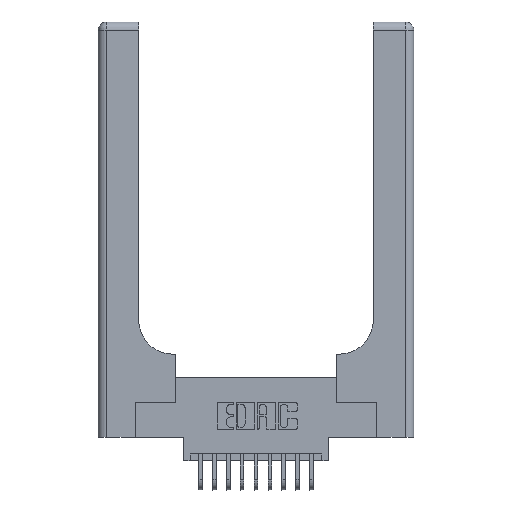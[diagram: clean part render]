
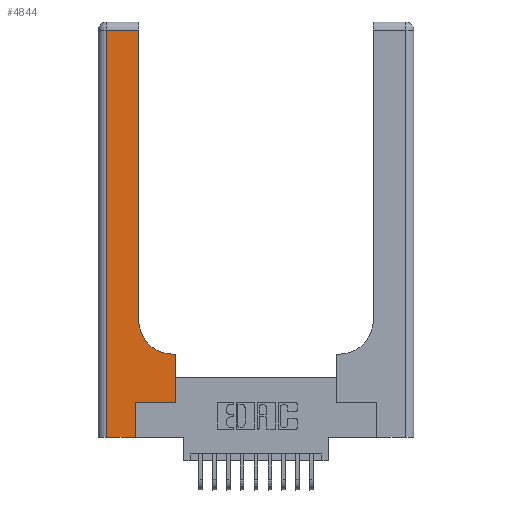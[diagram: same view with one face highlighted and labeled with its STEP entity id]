
A CAD part, top view. The second image highlights one B-rep face of the part: STEP entity #4844.
In plain terms, the highlighted planar face has unit normal (0, 0, 1).
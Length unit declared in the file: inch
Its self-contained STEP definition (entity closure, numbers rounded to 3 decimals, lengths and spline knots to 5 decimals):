
#27 = CARTESIAN_POINT ( 'NONE',  ( 0.2915, 2.94, 0.37 ) ) ;
#61 = DIRECTION ( 'NONE',  ( 0., 1., 0. ) ) ;
#300 = LINE ( 'NONE', #10796, #16571 ) ;
#415 = ORIENTED_EDGE ( 'NONE', *, *, #14892, .T. ) ;
#461 = DIRECTION ( 'NONE',  ( -1., 0., 0. ) ) ;
#616 = VECTOR ( 'NONE', #9260, 39.37008 ) ;
#671 = LINE ( 'NONE', #7835, #15627 ) ;
#719 = CARTESIAN_POINT ( 'NONE',  ( 0.5415, 0.6, 0.37 ) ) ;
#1242 = CARTESIAN_POINT ( 'NONE',  ( 0.269, 0., 0.37 ) ) ;
#1397 = CARTESIAN_POINT ( 'NONE',  ( 0.269, 0.25, 0.37 ) ) ;
#1563 = AXIS2_PLACEMENT_3D ( 'NONE', #11210, #4043, #2668 ) ;
#1673 = LINE ( 'NONE', #11323, #16840 ) ;
#1969 = CARTESIAN_POINT ( 'NONE',  ( 0.5585, 0.6, 0.37 ) ) ;
#2200 = DIRECTION ( 'NONE',  ( 0., 0., -1. ) ) ;
#2320 = CARTESIAN_POINT ( 'NONE',  ( 0.5415, 0.85, 0.37 ) ) ;
#2668 = DIRECTION ( 'NONE',  ( -1., 0., 0. ) ) ;
#2923 = CARTESIAN_POINT ( 'NONE',  ( 0.269, 0., 0.37 ) ) ;
#2958 = EDGE_CURVE ( 'NONE', #10657, #16845, #16515, .T. ) ;
#4043 = DIRECTION ( 'NONE',  ( 0., 0., -1. ) ) ;
#4255 = DIRECTION ( 'NONE',  ( -1., 0., 0. ) ) ;
#4281 = VERTEX_POINT ( 'NONE', #13822 ) ;
#4439 = LINE ( 'NONE', #8953, #616 ) ;
#4489 = ORIENTED_EDGE ( 'NONE', *, *, #18463, .T. ) ;
#4693 = LINE ( 'NONE', #1397, #8007 ) ;
#4844 = ADVANCED_FACE ( 'NONE', ( #7493 ), #15517, .F. ) ;
#5193 = DIRECTION ( 'NONE',  ( 1., 0., 0. ) ) ;
#5352 = VECTOR ( 'NONE', #461, 39.37008 ) ;
#5549 = CARTESIAN_POINT ( 'NONE',  ( 0.269, 0.25, 0.37 ) ) ;
#6067 = EDGE_CURVE ( 'NONE', #6499, #9241, #13495, .T. ) ;
#6171 = EDGE_LOOP ( 'NONE', ( #14357, #415, #17173, #10619, #13718, #17838, #4489, #11996, #8521 ) ) ;
#6417 = EDGE_CURVE ( 'NONE', #16845, #16767, #11688, .T. ) ;
#6499 = VERTEX_POINT ( 'NONE', #2923 ) ;
#7059 = VERTEX_POINT ( 'NONE', #16947 ) ;
#7493 = FACE_OUTER_BOUND ( 'NONE', #6171, .T. ) ;
#7745 = VECTOR ( 'NONE', #4255, 39.37008 ) ;
#7835 = CARTESIAN_POINT ( 'NONE',  ( 0., 0., 0.37 ) ) ;
#8007 = VECTOR ( 'NONE', #16933, 39.37008 ) ;
#8521 = ORIENTED_EDGE ( 'NONE', *, *, #6417, .T. ) ;
#8706 = CARTESIAN_POINT ( 'NONE',  ( 0.06, 2.94, 0.37 ) ) ;
#8884 = EDGE_CURVE ( 'NONE', #14968, #7059, #1673, .T. ) ;
#8953 = CARTESIAN_POINT ( 'NONE',  ( 0.2915, 3., 0.37 ) ) ;
#9241 = VERTEX_POINT ( 'NONE', #5549 ) ;
#9260 = DIRECTION ( 'NONE',  ( 0., 1., 0. ) ) ;
#10619 = ORIENTED_EDGE ( 'NONE', *, *, #11427, .T. ) ;
#10657 = VERTEX_POINT ( 'NONE', #1969 ) ;
#10796 = CARTESIAN_POINT ( 'NONE',  ( 0.5585, 0.25, 0.37 ) ) ;
#11210 = CARTESIAN_POINT ( 'NONE',  ( 0., 3., 0.37 ) ) ;
#11323 = CARTESIAN_POINT ( 'NONE',  ( 0.06, 3., 0.37 ) ) ;
#11427 = EDGE_CURVE ( 'NONE', #7059, #6499, #671, .T. ) ;
#11688 = CIRCLE ( 'NONE', #14840, 0.25 ) ;
#11996 = ORIENTED_EDGE ( 'NONE', *, *, #2958, .T. ) ;
#12262 = EDGE_CURVE ( 'NONE', #9241, #4281, #4693, .T. ) ;
#12531 = CARTESIAN_POINT ( 'NONE',  ( 0., 2.94, 0.37 ) ) ;
#12570 = VERTEX_POINT ( 'NONE', #27 ) ;
#13331 = EDGE_CURVE ( 'NONE', #16767, #12570, #4439, .T. ) ;
#13495 = LINE ( 'NONE', #1242, #17522 ) ;
#13718 = ORIENTED_EDGE ( 'NONE', *, *, #6067, .T. ) ;
#13822 = CARTESIAN_POINT ( 'NONE',  ( 0.5585, 0.25, 0.37 ) ) ;
#13823 = CARTESIAN_POINT ( 'NONE',  ( 0.2915, 0.85, 0.37 ) ) ;
#14249 = DIRECTION ( 'NONE',  ( 0., -1., 0. ) ) ;
#14357 = ORIENTED_EDGE ( 'NONE', *, *, #13331, .T. ) ;
#14457 = LINE ( 'NONE', #12531, #7745 ) ;
#14840 = AXIS2_PLACEMENT_3D ( 'NONE', #2320, #2200, #5193 ) ;
#14892 = EDGE_CURVE ( 'NONE', #12570, #14968, #14457, .T. ) ;
#14968 = VERTEX_POINT ( 'NONE', #8706 ) ;
#15517 = PLANE ( 'NONE',  #1563 ) ;
#15627 = VECTOR ( 'NONE', #16583, 39.37008 ) ;
#16515 = LINE ( 'NONE', #17560, #5352 ) ;
#16571 = VECTOR ( 'NONE', #18116, 39.37008 ) ;
#16583 = DIRECTION ( 'NONE',  ( 1., 0., 0. ) ) ;
#16767 = VERTEX_POINT ( 'NONE', #13823 ) ;
#16840 = VECTOR ( 'NONE', #14249, 39.37008 ) ;
#16845 = VERTEX_POINT ( 'NONE', #719 ) ;
#16933 = DIRECTION ( 'NONE',  ( 1., 0., 0. ) ) ;
#16947 = CARTESIAN_POINT ( 'NONE',  ( 0.06, 0., 0.37 ) ) ;
#17173 = ORIENTED_EDGE ( 'NONE', *, *, #8884, .T. ) ;
#17522 = VECTOR ( 'NONE', #61, 39.37008 ) ;
#17560 = CARTESIAN_POINT ( 'NONE',  ( 0.2915, 0.6, 0.37 ) ) ;
#17838 = ORIENTED_EDGE ( 'NONE', *, *, #12262, .T. ) ;
#18116 = DIRECTION ( 'NONE',  ( 0., 1., 0. ) ) ;
#18463 = EDGE_CURVE ( 'NONE', #4281, #10657, #300, .T. ) ;
